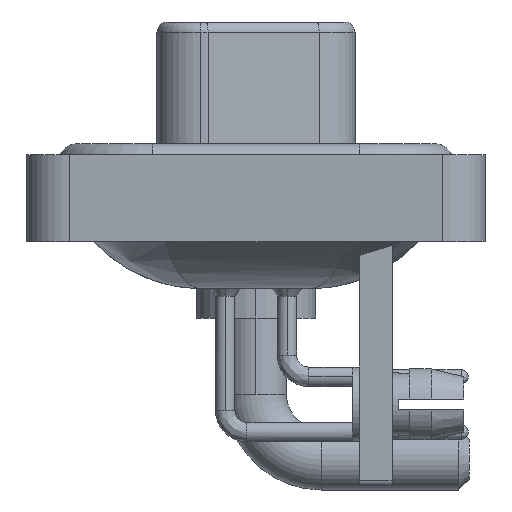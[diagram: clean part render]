
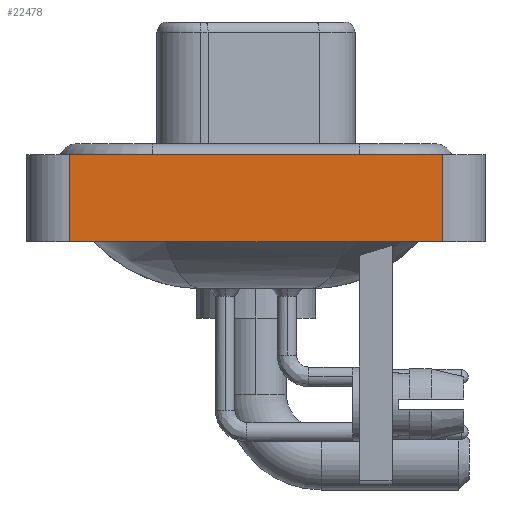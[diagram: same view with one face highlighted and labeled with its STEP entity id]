
A CAD part, left-side view. The second image highlights one B-rep face of the part: STEP entity #22478.
In plain terms, the highlighted planar face has unit normal (-1, 0, 0).
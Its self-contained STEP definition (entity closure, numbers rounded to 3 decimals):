
#2078 = CARTESIAN_POINT ( 'NONE',  ( -7.3, 8.55, -3.6 ) ) ;
#2122 = VECTOR ( 'NONE', #11401, 1000. ) ;
#2128 = EDGE_CURVE ( 'NONE', #22324, #16222, #21759, .T. ) ;
#3261 = CARTESIAN_POINT ( 'NONE',  ( -7.3, 8.55, -3.6 ) ) ;
#3280 = CARTESIAN_POINT ( 'NONE',  ( -7.3, -8.55, 0.4 ) ) ;
#4232 = CARTESIAN_POINT ( 'NONE',  ( -7.3, -8.55, 0.4 ) ) ;
#4741 = CARTESIAN_POINT ( 'NONE',  ( -7.3, 8.55, 0.4 ) ) ;
#7007 = AXIS2_PLACEMENT_3D ( 'NONE', #13282, #21921, #15033 ) ;
#11401 = DIRECTION ( 'NONE',  ( 0., 0., 1. ) ) ;
#12869 = FACE_OUTER_BOUND ( 'NONE', #15237, .T. ) ;
#13282 = CARTESIAN_POINT ( 'NONE',  ( -7.3, -8.55, -3.6 ) ) ;
#13478 = VERTEX_POINT ( 'NONE', #4232 ) ;
#13843 = CARTESIAN_POINT ( 'NONE',  ( -7.3, -8.55, -3.6 ) ) ;
#14406 = LINE ( 'NONE', #18582, #22758 ) ;
#14492 = ORIENTED_EDGE ( 'NONE', *, *, #2128, .F. ) ;
#15033 = DIRECTION ( 'NONE',  ( 0., 0., 1. ) ) ;
#15237 = EDGE_LOOP ( 'NONE', ( #21192, #15257, #14492, #24685 ) ) ;
#15257 = ORIENTED_EDGE ( 'NONE', *, *, #16618, .F. ) ;
#16222 = VERTEX_POINT ( 'NONE', #4741 ) ;
#16618 = EDGE_CURVE ( 'NONE', #16222, #13478, #22946, .T. ) ;
#17745 = VECTOR ( 'NONE', #23603, 1000. ) ;
#18582 = CARTESIAN_POINT ( 'NONE',  ( -7.3, -8.55, -3.6 ) ) ;
#20351 = VECTOR ( 'NONE', #23096, 1000. ) ;
#21192 = ORIENTED_EDGE ( 'NONE', *, *, #24339, .T. ) ;
#21759 = LINE ( 'NONE', #2078, #17745 ) ;
#21921 = DIRECTION ( 'NONE',  ( -1., 0., 0. ) ) ;
#22324 = VERTEX_POINT ( 'NONE', #3261 ) ;
#22478 = ADVANCED_FACE ( 'NONE', ( #12869 ), #26085, .T. ) ;
#22758 = VECTOR ( 'NONE', #27596, 1000. ) ;
#22946 = LINE ( 'NONE', #3280, #20351 ) ;
#23096 = DIRECTION ( 'NONE',  ( 0., -1., 0. ) ) ;
#23603 = DIRECTION ( 'NONE',  ( 0., 0., 1. ) ) ;
#24339 = EDGE_CURVE ( 'NONE', #25039, #13478, #26909, .T. ) ;
#24481 = EDGE_CURVE ( 'NONE', #22324, #25039, #14406, .T. ) ;
#24685 = ORIENTED_EDGE ( 'NONE', *, *, #24481, .T. ) ;
#25039 = VERTEX_POINT ( 'NONE', #27419 ) ;
#26085 = PLANE ( 'NONE',  #7007 ) ;
#26909 = LINE ( 'NONE', #13843, #2122 ) ;
#27419 = CARTESIAN_POINT ( 'NONE',  ( -7.3, -8.55, -3.6 ) ) ;
#27596 = DIRECTION ( 'NONE',  ( 0., -1., 0. ) ) ;
